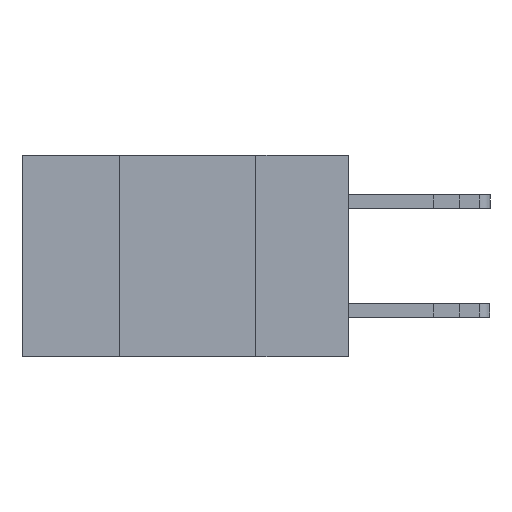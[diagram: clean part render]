
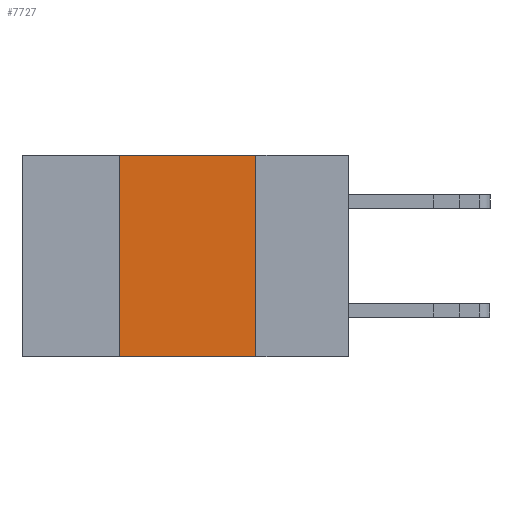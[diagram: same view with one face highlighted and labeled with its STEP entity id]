
A CAD part, left-side view. The second image highlights one B-rep face of the part: STEP entity #7727.
In plain terms, the highlighted planar face has unit normal (-1, 0, 0).
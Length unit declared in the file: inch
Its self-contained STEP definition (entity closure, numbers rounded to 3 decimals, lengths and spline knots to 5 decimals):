
#12 = ORIENTED_EDGE ( 'NONE', *, *, #8487, .F. ) ;
#130 = VERTEX_POINT ( 'NONE', #10566 ) ;
#270 = CARTESIAN_POINT ( 'NONE',  ( 0., 0.42, 0. ) ) ;
#295 = CARTESIAN_POINT ( 'NONE',  ( 0., 0.17, 0. ) ) ;
#371 = VERTEX_POINT ( 'NONE', #8485 ) ;
#539 = ORIENTED_EDGE ( 'NONE', *, *, #5225, .T. ) ;
#906 = CARTESIAN_POINT ( 'NONE',  ( 0., 0.42, -0.37 ) ) ;
#968 = FACE_OUTER_BOUND ( 'NONE', #1265, .T. ) ;
#1262 = DIRECTION ( 'NONE',  ( 0., 0., 1. ) ) ;
#1265 = EDGE_LOOP ( 'NONE', ( #4409, #11880, #12, #539 ) ) ;
#1737 = VECTOR ( 'NONE', #1828, 39.37008 ) ;
#1828 = DIRECTION ( 'NONE',  ( 0., -1., 0. ) ) ;
#2053 = CARTESIAN_POINT ( 'NONE',  ( 0., 0.6, 0. ) ) ;
#3602 = CARTESIAN_POINT ( 'NONE',  ( 0., 0.6, 0. ) ) ;
#3881 = LINE ( 'NONE', #3602, #1737 ) ;
#3891 = PLANE ( 'NONE',  #11669 ) ;
#4019 = EDGE_CURVE ( 'NONE', #7537, #130, #6194, .T. ) ;
#4409 = ORIENTED_EDGE ( 'NONE', *, *, #4019, .F. ) ;
#4837 = DIRECTION ( 'NONE',  ( 0., 0., -1. ) ) ;
#5225 = EDGE_CURVE ( 'NONE', #5277, #130, #5427, .T. ) ;
#5277 = VERTEX_POINT ( 'NONE', #906 ) ;
#5427 = LINE ( 'NONE', #9923, #10349 ) ;
#6194 = LINE ( 'NONE', #295, #10795 ) ;
#6609 = EDGE_CURVE ( 'NONE', #371, #7537, #3881, .T. ) ;
#7136 = CARTESIAN_POINT ( 'NONE',  ( 0., 0.17, 0. ) ) ;
#7537 = VERTEX_POINT ( 'NONE', #7136 ) ;
#7727 = ADVANCED_FACE ( 'NONE', ( #968 ), #3891, .F. ) ;
#8485 = CARTESIAN_POINT ( 'NONE',  ( 0., 0.42, 0. ) ) ;
#8487 = EDGE_CURVE ( 'NONE', #5277, #371, #9359, .T. ) ;
#9359 = LINE ( 'NONE', #270, #11448 ) ;
#9923 = CARTESIAN_POINT ( 'NONE',  ( 0., 0.6, -0.37 ) ) ;
#10349 = VECTOR ( 'NONE', #11007, 39.37008 ) ;
#10369 = DIRECTION ( 'NONE',  ( 1., 0., 0. ) ) ;
#10566 = CARTESIAN_POINT ( 'NONE',  ( 0., 0.17, -0.37 ) ) ;
#10795 = VECTOR ( 'NONE', #10887, 39.37008 ) ;
#10887 = DIRECTION ( 'NONE',  ( 0., 0., -1. ) ) ;
#11007 = DIRECTION ( 'NONE',  ( 0., -1., 0. ) ) ;
#11448 = VECTOR ( 'NONE', #1262, 39.37008 ) ;
#11669 = AXIS2_PLACEMENT_3D ( 'NONE', #2053, #10369, #4837 ) ;
#11880 = ORIENTED_EDGE ( 'NONE', *, *, #6609, .F. ) ;
